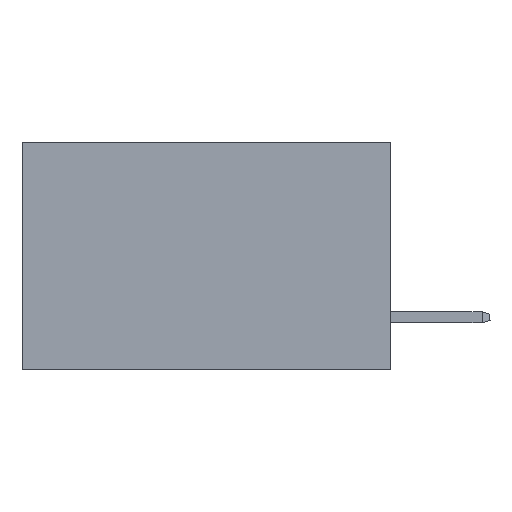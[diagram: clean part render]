
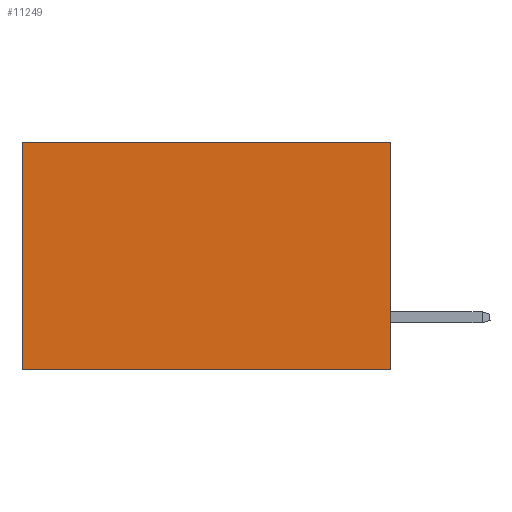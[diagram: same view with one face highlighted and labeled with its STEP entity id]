
A CAD part, left-side view. The second image highlights one B-rep face of the part: STEP entity #11249.
In plain terms, the highlighted planar face has unit normal (-1, 0, 0).
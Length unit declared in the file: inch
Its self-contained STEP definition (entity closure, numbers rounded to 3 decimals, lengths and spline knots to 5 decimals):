
#634 = VECTOR ( 'NONE', #6880, 39.37008 ) ;
#3365 = VECTOR ( 'NONE', #18491, 39.37008 ) ;
#3762 = CARTESIAN_POINT ( 'NONE',  ( 0.2875, 0., 0. ) ) ;
#4072 = DIRECTION ( 'NONE',  ( 0., 0., -1. ) ) ;
#4329 = CARTESIAN_POINT ( 'NONE',  ( 0.2875, 0., -0.37 ) ) ;
#4915 = LINE ( 'NONE', #8806, #3365 ) ;
#6528 = EDGE_CURVE ( 'NONE', #9761, #18433, #7326, .T. ) ;
#6880 = DIRECTION ( 'NONE',  ( 0., 1., 0. ) ) ;
#7326 = LINE ( 'NONE', #4329, #634 ) ;
#8129 = EDGE_CURVE ( 'NONE', #28906, #23485, #28967, .T. ) ;
#8806 = CARTESIAN_POINT ( 'NONE',  ( 0.2875, 0.6, 0. ) ) ;
#9761 = VERTEX_POINT ( 'NONE', #13021 ) ;
#10225 = EDGE_LOOP ( 'NONE', ( #17100, #24169, #14510, #19036 ) ) ;
#11249 = ADVANCED_FACE ( 'NONE', ( #16944 ), #26556, .F. ) ;
#11710 = CARTESIAN_POINT ( 'NONE',  ( 0.2875, 0.6, -0.37 ) ) ;
#12055 = CARTESIAN_POINT ( 'NONE',  ( 0.2875, 0., 0. ) ) ;
#12143 = AXIS2_PLACEMENT_3D ( 'NONE', #3762, #19085, #4072 ) ;
#12876 = EDGE_CURVE ( 'NONE', #23485, #18433, #4915, .T. ) ;
#13021 = CARTESIAN_POINT ( 'NONE',  ( 0.2875, 0., -0.37 ) ) ;
#14101 = DIRECTION ( 'NONE',  ( 0., 1., 0. ) ) ;
#14510 = ORIENTED_EDGE ( 'NONE', *, *, #24223, .F. ) ;
#16584 = LINE ( 'NONE', #12055, #25200 ) ;
#16888 = DIRECTION ( 'NONE',  ( 0., 0., -1. ) ) ;
#16944 = FACE_OUTER_BOUND ( 'NONE', #10225, .T. ) ;
#17100 = ORIENTED_EDGE ( 'NONE', *, *, #12876, .T. ) ;
#18433 = VERTEX_POINT ( 'NONE', #11710 ) ;
#18491 = DIRECTION ( 'NONE',  ( 0., 0., -1. ) ) ;
#19036 = ORIENTED_EDGE ( 'NONE', *, *, #8129, .T. ) ;
#19085 = DIRECTION ( 'NONE',  ( 1., 0., 0. ) ) ;
#21494 = CARTESIAN_POINT ( 'NONE',  ( 0.2875, 0., 0. ) ) ;
#23485 = VERTEX_POINT ( 'NONE', #32486 ) ;
#24169 = ORIENTED_EDGE ( 'NONE', *, *, #6528, .F. ) ;
#24223 = EDGE_CURVE ( 'NONE', #28906, #9761, #16584, .T. ) ;
#25200 = VECTOR ( 'NONE', #16888, 39.37008 ) ;
#26556 = PLANE ( 'NONE',  #12143 ) ;
#28186 = VECTOR ( 'NONE', #14101, 39.37008 ) ;
#28906 = VERTEX_POINT ( 'NONE', #21494 ) ;
#28967 = LINE ( 'NONE', #29141, #28186 ) ;
#29141 = CARTESIAN_POINT ( 'NONE',  ( 0.2875, 0., 0. ) ) ;
#32486 = CARTESIAN_POINT ( 'NONE',  ( 0.2875, 0.6, 0. ) ) ;
